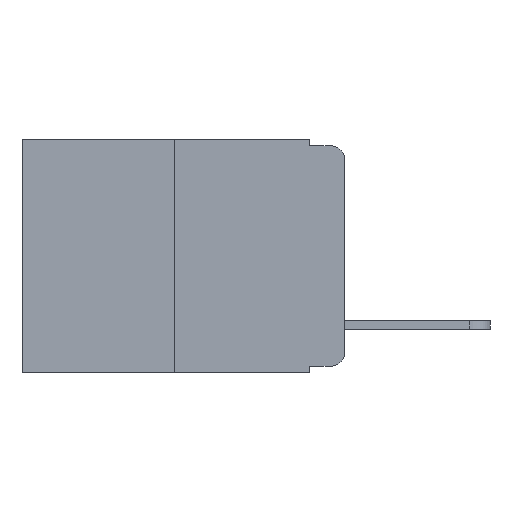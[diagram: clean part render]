
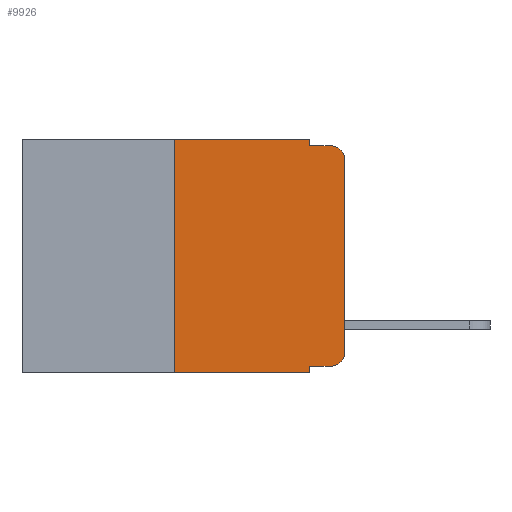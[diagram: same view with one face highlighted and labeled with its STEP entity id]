
A CAD part, left-side view. The second image highlights one B-rep face of the part: STEP entity #9926.
In plain terms, the highlighted planar face has unit normal (-1, 0, 0).
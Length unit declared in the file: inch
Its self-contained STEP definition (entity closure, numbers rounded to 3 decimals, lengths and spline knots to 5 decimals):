
#174 = VECTOR ( 'NONE', #11505, 39.37008 ) ;
#268 = CARTESIAN_POINT ( 'NONE',  ( 0., 0.051, -0.333 ) ) ;
#470 = DIRECTION ( 'NONE',  ( 0., -1., 0. ) ) ;
#675 = CARTESIAN_POINT ( 'NONE',  ( 0., 0.02, -0.333 ) ) ;
#836 = CARTESIAN_POINT ( 'NONE',  ( 0., 0.051, -0.343 ) ) ;
#869 = AXIS2_PLACEMENT_3D ( 'NONE', #8764, #14463, #8594 ) ;
#1388 = DIRECTION ( 'NONE',  ( 0., -1., 0. ) ) ;
#1483 = EDGE_CURVE ( 'NONE', #10449, #5411, #17729, .T. ) ;
#1517 = EDGE_CURVE ( 'NONE', #6792, #11435, #2453, .T. ) ;
#2140 = CIRCLE ( 'NONE', #14940, 0.02 ) ;
#2221 = VECTOR ( 'NONE', #7292, 39.37008 ) ;
#2453 = LINE ( 'NONE', #15783, #19792 ) ;
#2458 = LINE ( 'NONE', #8123, #19290 ) ;
#2467 = EDGE_CURVE ( 'NONE', #14815, #7380, #5127, .T. ) ;
#2494 = EDGE_CURVE ( 'NONE', #17518, #7380, #9724, .T. ) ;
#3721 = LINE ( 'NONE', #6113, #174 ) ;
#4909 = CARTESIAN_POINT ( 'NONE',  ( 0., 0.051, -0.01 ) ) ;
#5127 = CIRCLE ( 'NONE', #869, 0.02 ) ;
#5411 = VERTEX_POINT ( 'NONE', #836 ) ;
#5497 = VERTEX_POINT ( 'NONE', #675 ) ;
#6113 = CARTESIAN_POINT ( 'NONE',  ( 0., 0., 0. ) ) ;
#6792 = VERTEX_POINT ( 'NONE', #11026 ) ;
#7161 = DIRECTION ( 'NONE',  ( 1., 0., 0. ) ) ;
#7292 = DIRECTION ( 'NONE',  ( 0., -1., 0. ) ) ;
#7380 = VERTEX_POINT ( 'NONE', #13810 ) ;
#7646 = LINE ( 'NONE', #20078, #13612 ) ;
#7660 = FACE_OUTER_BOUND ( 'NONE', #17545, .T. ) ;
#7676 = EDGE_CURVE ( 'NONE', #5497, #8998, #2140, .T. ) ;
#7966 = DIRECTION ( 'NONE',  ( 0., 0., 1. ) ) ;
#8123 = CARTESIAN_POINT ( 'NONE',  ( 0., 0.051, 0. ) ) ;
#8584 = PLANE ( 'NONE',  #9736 ) ;
#8594 = DIRECTION ( 'NONE',  ( 0., 0., -1. ) ) ;
#8641 = VECTOR ( 'NONE', #1388, 39.37008 ) ;
#8764 = CARTESIAN_POINT ( 'NONE',  ( 0., 0.02, -0.03 ) ) ;
#8998 = VERTEX_POINT ( 'NONE', #21665 ) ;
#9678 = CARTESIAN_POINT ( 'NONE',  ( 0., 0.02, -0.313 ) ) ;
#9724 = LINE ( 'NONE', #4909, #8641 ) ;
#9736 = AXIS2_PLACEMENT_3D ( 'NONE', #20876, #7161, #15592 ) ;
#9926 = ADVANCED_FACE ( 'NONE', ( #7660 ), #8584, .F. ) ;
#10253 = VECTOR ( 'NONE', #12703, 39.37008 ) ;
#10449 = VERTEX_POINT ( 'NONE', #15884 ) ;
#11026 = CARTESIAN_POINT ( 'NONE',  ( 0., 0.25, 0. ) ) ;
#11435 = VERTEX_POINT ( 'NONE', #11572 ) ;
#11505 = DIRECTION ( 'NONE',  ( 0., 0., 1. ) ) ;
#11572 = CARTESIAN_POINT ( 'NONE',  ( 0., 0.051, 0. ) ) ;
#11884 = ORIENTED_EDGE ( 'NONE', *, *, #7676, .T. ) ;
#12585 = CARTESIAN_POINT ( 'NONE',  ( 0., 0.473, -0.343 ) ) ;
#12703 = DIRECTION ( 'NONE',  ( 0., 0., -1. ) ) ;
#12809 = DIRECTION ( 'NONE',  ( -1., 0., 0. ) ) ;
#12874 = CARTESIAN_POINT ( 'NONE',  ( 0., 0., -0.03 ) ) ;
#13121 = VECTOR ( 'NONE', #470, 39.37008 ) ;
#13260 = EDGE_CURVE ( 'NONE', #16345, #5411, #21648, .T. ) ;
#13612 = VECTOR ( 'NONE', #7966, 39.37008 ) ;
#13652 = LINE ( 'NONE', #268, #2221 ) ;
#13711 = ORIENTED_EDGE ( 'NONE', *, *, #1517, .F. ) ;
#13810 = CARTESIAN_POINT ( 'NONE',  ( 0., 0.02, -0.01 ) ) ;
#13961 = CARTESIAN_POINT ( 'NONE',  ( 0., 0.051, -0.01 ) ) ;
#14463 = DIRECTION ( 'NONE',  ( -1., 0., 0. ) ) ;
#14815 = VERTEX_POINT ( 'NONE', #12874 ) ;
#14935 = EDGE_CURVE ( 'NONE', #8998, #14815, #3721, .T. ) ;
#14940 = AXIS2_PLACEMENT_3D ( 'NONE', #9678, #12809, #20056 ) ;
#15388 = ORIENTED_EDGE ( 'NONE', *, *, #2467, .T. ) ;
#15592 = DIRECTION ( 'NONE',  ( 0., 0., -1. ) ) ;
#15783 = CARTESIAN_POINT ( 'NONE',  ( 0., 0.473, 0. ) ) ;
#15884 = CARTESIAN_POINT ( 'NONE',  ( 0., 0.25, -0.343 ) ) ;
#16345 = VERTEX_POINT ( 'NONE', #19070 ) ;
#16620 = ORIENTED_EDGE ( 'NONE', *, *, #20502, .F. ) ;
#16851 = DIRECTION ( 'NONE',  ( 0., 0., -1. ) ) ;
#17507 = DIRECTION ( 'NONE',  ( 0., -1., 0. ) ) ;
#17511 = ORIENTED_EDGE ( 'NONE', *, *, #1483, .T. ) ;
#17518 = VERTEX_POINT ( 'NONE', #13961 ) ;
#17545 = EDGE_LOOP ( 'NONE', ( #21256, #15388, #20495, #21901, #13711, #16620, #17511, #20559, #19233, #11884 ) ) ;
#17729 = LINE ( 'NONE', #12585, #13121 ) ;
#19070 = CARTESIAN_POINT ( 'NONE',  ( 0., 0.051, -0.333 ) ) ;
#19233 = ORIENTED_EDGE ( 'NONE', *, *, #19741, .T. ) ;
#19290 = VECTOR ( 'NONE', #16851, 39.37008 ) ;
#19741 = EDGE_CURVE ( 'NONE', #16345, #5497, #13652, .T. ) ;
#19792 = VECTOR ( 'NONE', #17507, 39.37008 ) ;
#19868 = CARTESIAN_POINT ( 'NONE',  ( 0., 0.051, 0. ) ) ;
#20056 = DIRECTION ( 'NONE',  ( 0., 0., -1. ) ) ;
#20078 = CARTESIAN_POINT ( 'NONE',  ( 0., 0.25, 0. ) ) ;
#20495 = ORIENTED_EDGE ( 'NONE', *, *, #2494, .F. ) ;
#20502 = EDGE_CURVE ( 'NONE', #10449, #6792, #7646, .T. ) ;
#20544 = EDGE_CURVE ( 'NONE', #11435, #17518, #2458, .T. ) ;
#20559 = ORIENTED_EDGE ( 'NONE', *, *, #13260, .F. ) ;
#20876 = CARTESIAN_POINT ( 'NONE',  ( 0., 0.473, 0. ) ) ;
#21256 = ORIENTED_EDGE ( 'NONE', *, *, #14935, .T. ) ;
#21648 = LINE ( 'NONE', #19868, #10253 ) ;
#21665 = CARTESIAN_POINT ( 'NONE',  ( 0., 0., -0.313 ) ) ;
#21901 = ORIENTED_EDGE ( 'NONE', *, *, #20544, .F. ) ;
